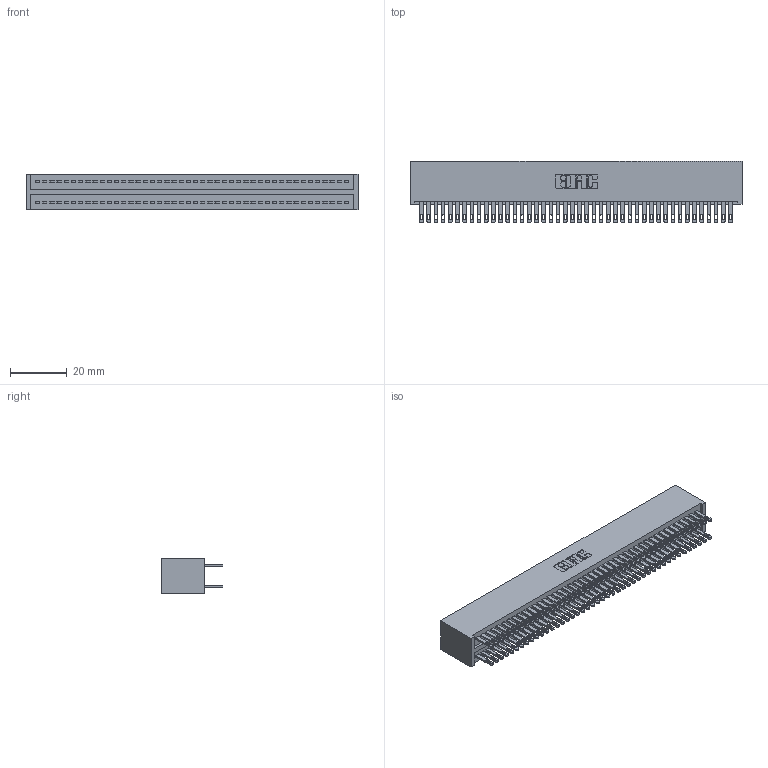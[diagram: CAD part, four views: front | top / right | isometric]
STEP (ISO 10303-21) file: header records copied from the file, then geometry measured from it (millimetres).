
FILE_DESCRIPTION (( 'STEP AP203' ), '1' );
FILE_NAME ('325-088-500-201.STEP', '2020-02-25T05:20:49', ( '' ), ( '' ), 'SwSTEP 2.0', 'SolidWorks 2016', '' );
FILE_SCHEMA (( 'CONFIG_CONTROL_DESIGN' ));
Length unit declared in the file: inch
Products named in the file (3): 325-088-500-201; 325-292-001_325-293-100; 325 Part_Lugless
Assembly tree (89 placements, depth 2):
  325-088-500-201
    325 Part_Lugless
    325-292-001_325-293-100  x88
Bounding box: 117.4 x 21.84 x 12.45 mm (x, y, z)
Volume: 16048.7 mm3; surface area: 21053.4 mm2
Topology: 89 solids, 89 shells, 4330 faces, 13223 edges, 8814 vertices
Faces by surface type: plane 2706, cylinder 1624
Entity records: 27701 total; most frequent: CARTESIAN_POINT 4586, ORIENTED_EDGE 4522, DIRECTION 3909, EDGE_CURVE 2261, VECTOR 2137, LINE 2137, VERTEX_POINT 1506, AXIS2_PLACEMENT_3D 886
